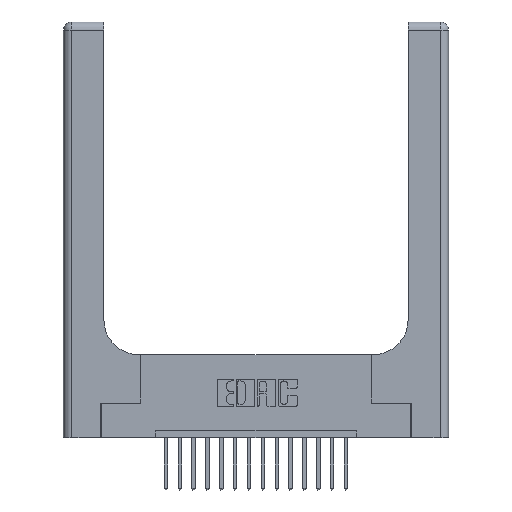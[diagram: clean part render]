
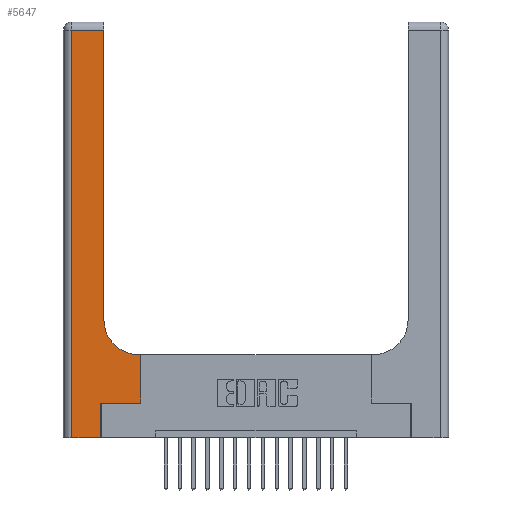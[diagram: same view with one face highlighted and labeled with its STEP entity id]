
A CAD part, top view. The second image highlights one B-rep face of the part: STEP entity #5647.
In plain terms, the highlighted planar face has unit normal (0, 0, 1).
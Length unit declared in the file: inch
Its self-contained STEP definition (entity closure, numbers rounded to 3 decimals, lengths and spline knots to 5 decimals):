
#613 = EDGE_CURVE ( 'NONE', #18749, #2755, #5682, .T. ) ;
#806 = DIRECTION ( 'NONE',  ( 1., 0., 0. ) ) ;
#1020 = DIRECTION ( 'NONE',  ( 0., 0., -1. ) ) ;
#1224 = AXIS2_PLACEMENT_3D ( 'NONE', #15961, #1020, #8737 ) ;
#1682 = LINE ( 'NONE', #2638, #8768 ) ;
#2415 = LINE ( 'NONE', #13659, #17239 ) ;
#2417 = CARTESIAN_POINT ( 'NONE',  ( 0.06, 0., 0.37 ) ) ;
#2508 = ORIENTED_EDGE ( 'NONE', *, *, #8585, .T. ) ;
#2638 = CARTESIAN_POINT ( 'NONE',  ( 0.2915, 0.6, 0.37 ) ) ;
#2704 = EDGE_CURVE ( 'NONE', #2755, #9551, #14554, .T. ) ;
#2731 = CARTESIAN_POINT ( 'NONE',  ( 0.269, 0.25, 0.37 ) ) ;
#2755 = VERTEX_POINT ( 'NONE', #18975 ) ;
#2976 = PLANE ( 'NONE',  #14086 ) ;
#4053 = DIRECTION ( 'NONE',  ( -1., 0., 0. ) ) ;
#4680 = DIRECTION ( 'NONE',  ( 1., 0., 0. ) ) ;
#4706 = ORIENTED_EDGE ( 'NONE', *, *, #2704, .T. ) ;
#5348 = CARTESIAN_POINT ( 'NONE',  ( 0.2915, 0.85, 0.37 ) ) ;
#5647 = ADVANCED_FACE ( 'NONE', ( #12544 ), #2976, .F. ) ;
#5682 = LINE ( 'NONE', #17060, #6489 ) ;
#6025 = VECTOR ( 'NONE', #8103, 39.37008 ) ;
#6060 = VECTOR ( 'NONE', #11239, 39.37008 ) ;
#6487 = VERTEX_POINT ( 'NONE', #5348 ) ;
#6489 = VECTOR ( 'NONE', #806, 39.37008 ) ;
#6517 = ORIENTED_EDGE ( 'NONE', *, *, #12874, .T. ) ;
#6785 = EDGE_CURVE ( 'NONE', #15135, #9126, #11067, .T. ) ;
#6806 = VERTEX_POINT ( 'NONE', #11764 ) ;
#7437 = LINE ( 'NONE', #15676, #6025 ) ;
#8103 = DIRECTION ( 'NONE',  ( 0., 1., 0. ) ) ;
#8135 = CARTESIAN_POINT ( 'NONE',  ( 0., 2.94, 0.37 ) ) ;
#8357 = VERTEX_POINT ( 'NONE', #2417 ) ;
#8585 = EDGE_CURVE ( 'NONE', #8357, #6806, #14072, .T. ) ;
#8737 = DIRECTION ( 'NONE',  ( 1., 0., 0. ) ) ;
#8768 = VECTOR ( 'NONE', #4053, 39.37008 ) ;
#8908 = ORIENTED_EDGE ( 'NONE', *, *, #9464, .T. ) ;
#9070 = ORIENTED_EDGE ( 'NONE', *, *, #613, .T. ) ;
#9126 = VERTEX_POINT ( 'NONE', #11823 ) ;
#9301 = EDGE_CURVE ( 'NONE', #6487, #15135, #7437, .T. ) ;
#9464 = EDGE_CURVE ( 'NONE', #12016, #6487, #11905, .T. ) ;
#9551 = VERTEX_POINT ( 'NONE', #13613 ) ;
#10287 = ORIENTED_EDGE ( 'NONE', *, *, #15277, .T. ) ;
#10584 = ORIENTED_EDGE ( 'NONE', *, *, #14836, .T. ) ;
#10855 = LINE ( 'NONE', #19081, #16943 ) ;
#11067 = LINE ( 'NONE', #8135, #15083 ) ;
#11239 = DIRECTION ( 'NONE',  ( 0., 1., 0. ) ) ;
#11764 = CARTESIAN_POINT ( 'NONE',  ( 0.269, 0., 0.37 ) ) ;
#11823 = CARTESIAN_POINT ( 'NONE',  ( 0.06, 2.94, 0.37 ) ) ;
#11905 = CIRCLE ( 'NONE', #1224, 0.25 ) ;
#12016 = VERTEX_POINT ( 'NONE', #16802 ) ;
#12544 = FACE_OUTER_BOUND ( 'NONE', #14449, .T. ) ;
#12548 = ORIENTED_EDGE ( 'NONE', *, *, #6785, .T. ) ;
#12850 = ORIENTED_EDGE ( 'NONE', *, *, #9301, .T. ) ;
#12874 = EDGE_CURVE ( 'NONE', #9126, #8357, #10855, .T. ) ;
#12893 = CARTESIAN_POINT ( 'NONE',  ( 0.5585, 0.25, 0.37 ) ) ;
#13132 = VECTOR ( 'NONE', #4680, 39.37008 ) ;
#13613 = CARTESIAN_POINT ( 'NONE',  ( 0.5585, 0.6, 0.37 ) ) ;
#13659 = CARTESIAN_POINT ( 'NONE',  ( 0.269, 0., 0.37 ) ) ;
#14072 = LINE ( 'NONE', #16425, #13132 ) ;
#14086 = AXIS2_PLACEMENT_3D ( 'NONE', #16057, #15050, #16513 ) ;
#14449 = EDGE_LOOP ( 'NONE', ( #12850, #12548, #6517, #2508, #10584, #9070, #4706, #10287, #8908 ) ) ;
#14554 = LINE ( 'NONE', #12893, #6060 ) ;
#14836 = EDGE_CURVE ( 'NONE', #6806, #18749, #2415, .T. ) ;
#15050 = DIRECTION ( 'NONE',  ( 0., 0., -1. ) ) ;
#15083 = VECTOR ( 'NONE', #19238, 39.37008 ) ;
#15135 = VERTEX_POINT ( 'NONE', #18680 ) ;
#15277 = EDGE_CURVE ( 'NONE', #9551, #12016, #1682, .T. ) ;
#15676 = CARTESIAN_POINT ( 'NONE',  ( 0.2915, 3., 0.37 ) ) ;
#15961 = CARTESIAN_POINT ( 'NONE',  ( 0.5415, 0.85, 0.37 ) ) ;
#16057 = CARTESIAN_POINT ( 'NONE',  ( 0., 3., 0.37 ) ) ;
#16425 = CARTESIAN_POINT ( 'NONE',  ( 0., 0., 0.37 ) ) ;
#16513 = DIRECTION ( 'NONE',  ( -1., 0., 0. ) ) ;
#16802 = CARTESIAN_POINT ( 'NONE',  ( 0.5415, 0.6, 0.37 ) ) ;
#16943 = VECTOR ( 'NONE', #17362, 39.37008 ) ;
#17060 = CARTESIAN_POINT ( 'NONE',  ( 0.269, 0.25, 0.37 ) ) ;
#17239 = VECTOR ( 'NONE', #17495, 39.37008 ) ;
#17362 = DIRECTION ( 'NONE',  ( 0., -1., 0. ) ) ;
#17495 = DIRECTION ( 'NONE',  ( 0., 1., 0. ) ) ;
#18680 = CARTESIAN_POINT ( 'NONE',  ( 0.2915, 2.94, 0.37 ) ) ;
#18749 = VERTEX_POINT ( 'NONE', #2731 ) ;
#18975 = CARTESIAN_POINT ( 'NONE',  ( 0.5585, 0.25, 0.37 ) ) ;
#19081 = CARTESIAN_POINT ( 'NONE',  ( 0.06, 3., 0.37 ) ) ;
#19238 = DIRECTION ( 'NONE',  ( -1., 0., 0. ) ) ;
